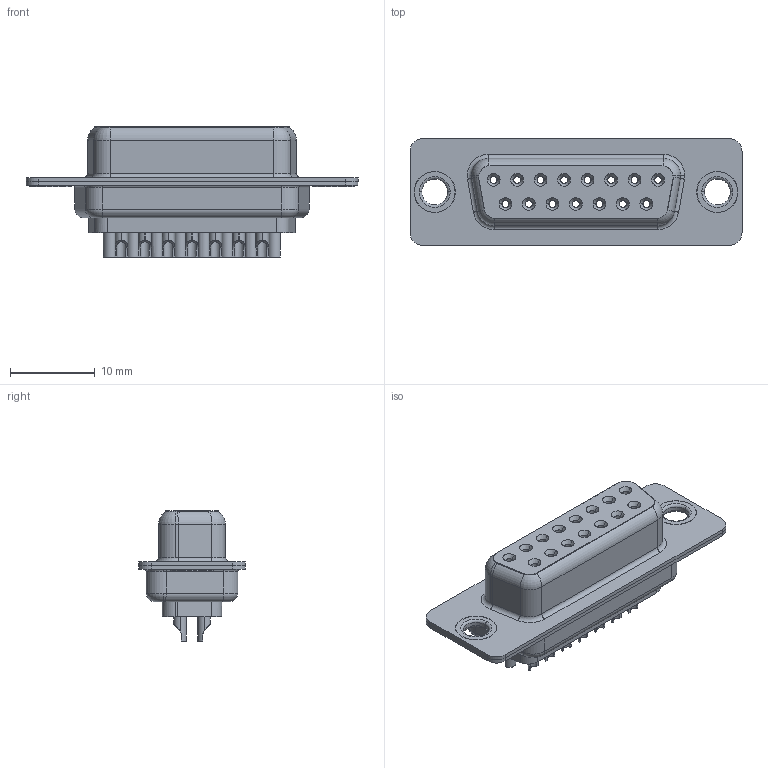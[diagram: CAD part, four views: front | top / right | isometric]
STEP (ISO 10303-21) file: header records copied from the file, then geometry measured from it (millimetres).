
FILE_DESCRIPTION (( 'STEP AP203' ), '1' );
FILE_NAME ('628-015-322-041.STEP', '2020-07-14T01:35:36', ( '' ), ( '' ), 'SwSTEP 2.0', 'SolidWorks 2020', '' );
FILE_SCHEMA (( 'CONFIG_CONTROL_DESIGN' ));
Length unit declared in the file: millimetre
Products named in the file (7): 628-015-322-041; 628 Contact Row 1_22L; 628 Contact Row 2_22L; 628 Shell Rear_15 Contacts; 628 Shell Front_15 Contacts; 628 Housing_15 LP; 628 Thru Hole Rivet
Assembly tree (20 placements, depth 2):
  628-015-322-041
    628 Housing_15 LP
    628 Shell Front_15 Contacts
    628 Shell Rear_15 Contacts
    628 Contact Row 1_22L  x8
    628 Contact Row 2_22L  x7
    628 Thru Hole Rivet  x2
Bounding box: 39.15 x 12.6 x 15.35 mm (x, y, z)
Volume: 2470 mm3; surface area: 6208.7 mm2
Topology: 20 solids, 20 shells, 1588 faces, 3993 edges, 2501 vertices
Faces by surface type: cylinder 496, plane 382, torus 335, bspline 300, cone 75
Entity records: 19653 total; most frequent: CARTESIAN_POINT 4947, DIRECTION 2991, ORIENTED_EDGE 2758, EDGE_CURVE 1379, AXIS2_PLACEMENT_3D 1248, VERTEX_POINT 865, CIRCLE 685, EDGE_LOOP 678
